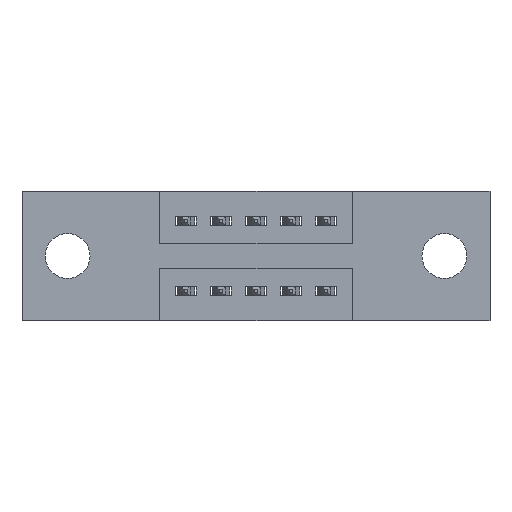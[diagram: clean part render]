
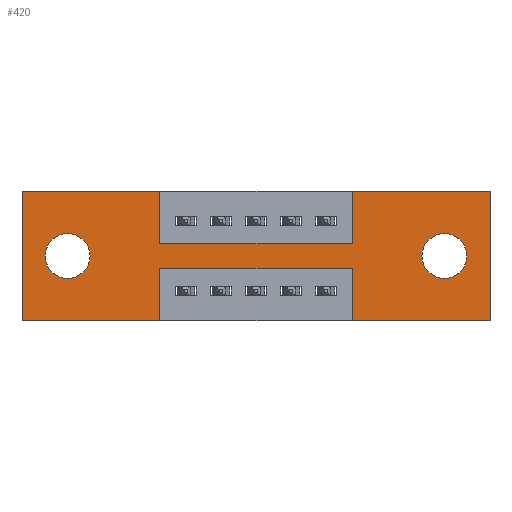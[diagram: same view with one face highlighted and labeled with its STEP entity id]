
A CAD part, front view. The second image highlights one B-rep face of the part: STEP entity #420.
In plain terms, the highlighted planar face has unit normal (0, -1, 0).
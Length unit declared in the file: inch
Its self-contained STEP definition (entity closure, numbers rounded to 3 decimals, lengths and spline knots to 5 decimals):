
#195 = VECTOR ( 'NONE', #7719, 39.37008 ) ;
#223 = CARTESIAN_POINT ( 'NONE',  ( 1.205, 0., -0.249 ) ) ;
#349 = CIRCLE ( 'NONE', #5446, 0.064 ) ;
#384 = CARTESIAN_POINT ( 'NONE',  ( 0.3925, 0., -0.15 ) ) ;
#420 = ADVANCED_FACE ( 'NONE', ( #4459, #6033, #7854 ), #3960, .T. ) ;
#509 = CARTESIAN_POINT ( 'NONE',  ( 0.3925, 0., -0.37 ) ) ;
#520 = DIRECTION ( 'NONE',  ( 0., 0., -1. ) ) ;
#557 = VERTEX_POINT ( 'NONE', #2503 ) ;
#654 = LINE ( 'NONE', #4079, #5937 ) ;
#726 = LINE ( 'NONE', #7201, #2037 ) ;
#905 = CARTESIAN_POINT ( 'NONE',  ( 0.9425, 0., 0. ) ) ;
#1037 = EDGE_LOOP ( 'NONE', ( #2748, #1244 ) ) ;
#1180 = VERTEX_POINT ( 'NONE', #8054 ) ;
#1244 = ORIENTED_EDGE ( 'NONE', *, *, #5568, .T. ) ;
#1255 = DIRECTION ( 'NONE',  ( 0., 0., 1. ) ) ;
#1366 = DIRECTION ( 'NONE',  ( -1., 0., 0. ) ) ;
#1380 = ORIENTED_EDGE ( 'NONE', *, *, #6455, .F. ) ;
#1432 = CARTESIAN_POINT ( 'NONE',  ( 1.335, 0., -0.37 ) ) ;
#1447 = CARTESIAN_POINT ( 'NONE',  ( 0.3925, 0., -0.22 ) ) ;
#1555 = VECTOR ( 'NONE', #520, 39.37008 ) ;
#1600 = DIRECTION ( 'NONE',  ( -1., 0., 0. ) ) ;
#1616 = ORIENTED_EDGE ( 'NONE', *, *, #3024, .F. ) ;
#1623 = CARTESIAN_POINT ( 'NONE',  ( 0., 0., -0.37 ) ) ;
#1661 = DIRECTION ( 'NONE',  ( -1., 0., 0. ) ) ;
#1762 = DIRECTION ( 'NONE',  ( 0., 1., 0. ) ) ;
#1829 = EDGE_CURVE ( 'NONE', #8554, #4874, #349, .T. ) ;
#1997 = CARTESIAN_POINT ( 'NONE',  ( 1.205, 0., -0.185 ) ) ;
#2001 = EDGE_CURVE ( 'NONE', #3961, #4369, #2046, .T. ) ;
#2029 = CARTESIAN_POINT ( 'NONE',  ( 0.9425, 0., -0.37 ) ) ;
#2037 = VECTOR ( 'NONE', #7103, 39.37008 ) ;
#2042 = CIRCLE ( 'NONE', #5236, 0.064 ) ;
#2046 = LINE ( 'NONE', #1447, #8512 ) ;
#2261 = EDGE_CURVE ( 'NONE', #557, #3036, #7384, .T. ) ;
#2264 = EDGE_CURVE ( 'NONE', #3876, #557, #726, .T. ) ;
#2503 = CARTESIAN_POINT ( 'NONE',  ( 0., 0., 0. ) ) ;
#2504 = CARTESIAN_POINT ( 'NONE',  ( 0.9425, 0., -0.22 ) ) ;
#2511 = CARTESIAN_POINT ( 'NONE',  ( 0.9425, 0., 0. ) ) ;
#2588 = CARTESIAN_POINT ( 'NONE',  ( 0.3925, 0., 0. ) ) ;
#2648 = CARTESIAN_POINT ( 'NONE',  ( 0., 0., -0.37 ) ) ;
#2654 = ORIENTED_EDGE ( 'NONE', *, *, #2264, .F. ) ;
#2747 = DIRECTION ( 'NONE',  ( 0., 0., -1. ) ) ;
#2748 = ORIENTED_EDGE ( 'NONE', *, *, #6971, .T. ) ;
#3024 = EDGE_CURVE ( 'NONE', #6989, #5884, #8783, .T. ) ;
#3036 = VERTEX_POINT ( 'NONE', #6911 ) ;
#3039 = EDGE_LOOP ( 'NONE', ( #5492, #7523, #7940, #8131, #1380, #1616, #5391, #3154, #3340, #5916, #2654, #3060 ) ) ;
#3060 = ORIENTED_EDGE ( 'NONE', *, *, #4081, .F. ) ;
#3154 = ORIENTED_EDGE ( 'NONE', *, *, #3530, .F. ) ;
#3233 = DIRECTION ( 'NONE',  ( 0., 0., -1. ) ) ;
#3266 = CIRCLE ( 'NONE', #6509, 0.064 ) ;
#3297 = VECTOR ( 'NONE', #4074, 39.37008 ) ;
#3301 = VECTOR ( 'NONE', #7136, 39.37008 ) ;
#3330 = ORIENTED_EDGE ( 'NONE', *, *, #5571, .T. ) ;
#3340 = ORIENTED_EDGE ( 'NONE', *, *, #8590, .F. ) ;
#3352 = DIRECTION ( 'NONE',  ( 0., 0., -1. ) ) ;
#3366 = CARTESIAN_POINT ( 'NONE',  ( 0.13, 0., -0.185 ) ) ;
#3530 = EDGE_CURVE ( 'NONE', #6409, #1180, #8584, .T. ) ;
#3876 = VERTEX_POINT ( 'NONE', #2648 ) ;
#3960 = PLANE ( 'NONE',  #7308 ) ;
#3961 = VERTEX_POINT ( 'NONE', #2504 ) ;
#4028 = DIRECTION ( 'NONE',  ( 0., 0., 1. ) ) ;
#4074 = DIRECTION ( 'NONE',  ( 1., 0., 0. ) ) ;
#4079 = CARTESIAN_POINT ( 'NONE',  ( 0., 0., -0.37 ) ) ;
#4081 = EDGE_CURVE ( 'NONE', #5670, #3876, #6851, .T. ) ;
#4090 = CARTESIAN_POINT ( 'NONE',  ( 0.3925, 0., -0.15 ) ) ;
#4156 = CARTESIAN_POINT ( 'NONE',  ( 0., 0., -0.37 ) ) ;
#4249 = EDGE_CURVE ( 'NONE', #4369, #5670, #5120, .T. ) ;
#4341 = DIRECTION ( 'NONE',  ( 0., 0., 1. ) ) ;
#4361 = DIRECTION ( 'NONE',  ( 0., 1., 0. ) ) ;
#4369 = VERTEX_POINT ( 'NONE', #6541 ) ;
#4375 = VERTEX_POINT ( 'NONE', #223 ) ;
#4378 = CARTESIAN_POINT ( 'NONE',  ( 0.13, 0., -0.185 ) ) ;
#4459 = FACE_BOUND ( 'NONE', #1037, .T. ) ;
#4649 = CARTESIAN_POINT ( 'NONE',  ( 1.335, 0., 0. ) ) ;
#4842 = LINE ( 'NONE', #7869, #6463 ) ;
#4874 = VERTEX_POINT ( 'NONE', #5848 ) ;
#4945 = VECTOR ( 'NONE', #3352, 39.37008 ) ;
#5120 = LINE ( 'NONE', #509, #1555 ) ;
#5236 = AXIS2_PLACEMENT_3D ( 'NONE', #5753, #1762, #6478 ) ;
#5290 = EDGE_CURVE ( 'NONE', #1180, #6989, #8451, .T. ) ;
#5343 = EDGE_LOOP ( 'NONE', ( #3330, #6898 ) ) ;
#5391 = ORIENTED_EDGE ( 'NONE', *, *, #5290, .F. ) ;
#5446 = AXIS2_PLACEMENT_3D ( 'NONE', #4378, #4361, #4341 ) ;
#5492 = ORIENTED_EDGE ( 'NONE', *, *, #4249, .F. ) ;
#5568 = EDGE_CURVE ( 'NONE', #4375, #6940, #3266, .T. ) ;
#5571 = EDGE_CURVE ( 'NONE', #4874, #8554, #8352, .T. ) ;
#5670 = VERTEX_POINT ( 'NONE', #8094 ) ;
#5673 = EDGE_CURVE ( 'NONE', #5769, #8139, #654, .T. ) ;
#5753 = CARTESIAN_POINT ( 'NONE',  ( 1.205, 0., -0.185 ) ) ;
#5769 = VERTEX_POINT ( 'NONE', #1432 ) ;
#5848 = CARTESIAN_POINT ( 'NONE',  ( 0.13, 0., -0.121 ) ) ;
#5884 = VERTEX_POINT ( 'NONE', #8890 ) ;
#5916 = ORIENTED_EDGE ( 'NONE', *, *, #2261, .F. ) ;
#5937 = VECTOR ( 'NONE', #1366, 39.37008 ) ;
#5977 = DIRECTION ( 'NONE',  ( 0., -1., 0. ) ) ;
#6033 = FACE_BOUND ( 'NONE', #5343, .T. ) ;
#6204 = EDGE_CURVE ( 'NONE', #8139, #3961, #4842, .T. ) ;
#6409 = VERTEX_POINT ( 'NONE', #384 ) ;
#6432 = VECTOR ( 'NONE', #3233, 39.37008 ) ;
#6455 = EDGE_CURVE ( 'NONE', #5884, #5769, #8709, .T. ) ;
#6463 = VECTOR ( 'NONE', #8494, 39.37008 ) ;
#6478 = DIRECTION ( 'NONE',  ( 0., 0., -1. ) ) ;
#6509 = AXIS2_PLACEMENT_3D ( 'NONE', #1997, #6721, #2747 ) ;
#6521 = CARTESIAN_POINT ( 'NONE',  ( 0.13, 0., -0.249 ) ) ;
#6541 = CARTESIAN_POINT ( 'NONE',  ( 0.3925, 0., -0.22 ) ) ;
#6647 = VECTOR ( 'NONE', #1600, 39.37008 ) ;
#6670 = LINE ( 'NONE', #2588, #6432 ) ;
#6721 = DIRECTION ( 'NONE',  ( 0., 1., 0. ) ) ;
#6729 = VECTOR ( 'NONE', #1255, 39.37008 ) ;
#6851 = LINE ( 'NONE', #1623, #6647 ) ;
#6898 = ORIENTED_EDGE ( 'NONE', *, *, #1829, .T. ) ;
#6911 = CARTESIAN_POINT ( 'NONE',  ( 0.3925, 0., 0. ) ) ;
#6940 = VERTEX_POINT ( 'NONE', #8401 ) ;
#6971 = EDGE_CURVE ( 'NONE', #6940, #4375, #2042, .T. ) ;
#6972 = AXIS2_PLACEMENT_3D ( 'NONE', #3366, #8046, #4028 ) ;
#6989 = VERTEX_POINT ( 'NONE', #2511 ) ;
#7103 = DIRECTION ( 'NONE',  ( 0., 0., 1. ) ) ;
#7136 = DIRECTION ( 'NONE',  ( 1., 0., 0. ) ) ;
#7162 = CARTESIAN_POINT ( 'NONE',  ( 0., 0., 0. ) ) ;
#7201 = CARTESIAN_POINT ( 'NONE',  ( 0., 0., 0. ) ) ;
#7260 = CARTESIAN_POINT ( 'NONE',  ( 0., 0., 0. ) ) ;
#7308 = AXIS2_PLACEMENT_3D ( 'NONE', #4156, #5977, #7606 ) ;
#7384 = LINE ( 'NONE', #7260, #195 ) ;
#7523 = ORIENTED_EDGE ( 'NONE', *, *, #2001, .F. ) ;
#7606 = DIRECTION ( 'NONE',  ( 0., 0., -1. ) ) ;
#7719 = DIRECTION ( 'NONE',  ( 1., 0., 0. ) ) ;
#7854 = FACE_OUTER_BOUND ( 'NONE', #3039, .T. ) ;
#7869 = CARTESIAN_POINT ( 'NONE',  ( 0.9425, 0., -0.37 ) ) ;
#7940 = ORIENTED_EDGE ( 'NONE', *, *, #6204, .F. ) ;
#8046 = DIRECTION ( 'NONE',  ( 0., 1., 0. ) ) ;
#8054 = CARTESIAN_POINT ( 'NONE',  ( 0.9425, 0., -0.15 ) ) ;
#8094 = CARTESIAN_POINT ( 'NONE',  ( 0.3925, 0., -0.37 ) ) ;
#8131 = ORIENTED_EDGE ( 'NONE', *, *, #5673, .F. ) ;
#8139 = VERTEX_POINT ( 'NONE', #2029 ) ;
#8352 = CIRCLE ( 'NONE', #6972, 0.064 ) ;
#8401 = CARTESIAN_POINT ( 'NONE',  ( 1.205, 0., -0.121 ) ) ;
#8451 = LINE ( 'NONE', #905, #6729 ) ;
#8494 = DIRECTION ( 'NONE',  ( 0., 0., 1. ) ) ;
#8512 = VECTOR ( 'NONE', #1661, 39.37008 ) ;
#8554 = VERTEX_POINT ( 'NONE', #6521 ) ;
#8584 = LINE ( 'NONE', #4090, #3297 ) ;
#8590 = EDGE_CURVE ( 'NONE', #3036, #6409, #6670, .T. ) ;
#8709 = LINE ( 'NONE', #4649, #4945 ) ;
#8783 = LINE ( 'NONE', #7162, #3301 ) ;
#8890 = CARTESIAN_POINT ( 'NONE',  ( 1.335, 0., 0. ) ) ;
